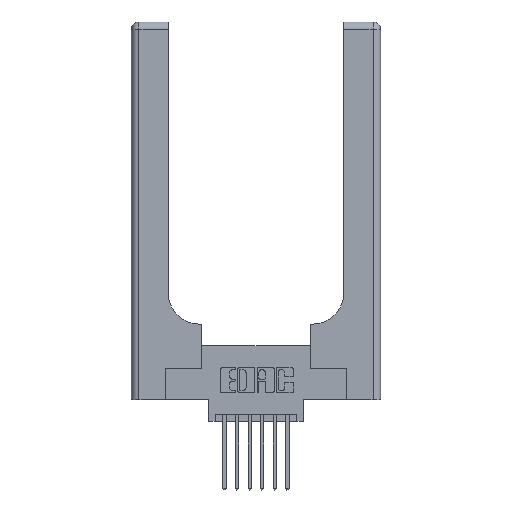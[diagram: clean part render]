
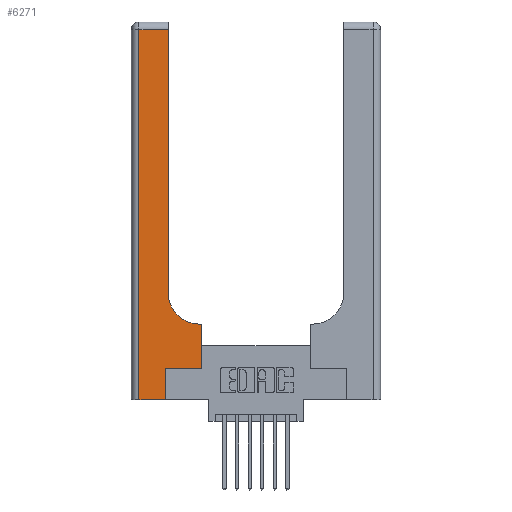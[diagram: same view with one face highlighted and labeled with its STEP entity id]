
A CAD part, top view. The second image highlights one B-rep face of the part: STEP entity #6271.
In plain terms, the highlighted planar face has unit normal (0, 0, 1).
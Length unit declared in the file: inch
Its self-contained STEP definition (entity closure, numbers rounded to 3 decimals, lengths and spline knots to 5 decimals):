
#11 = DIRECTION ( 'NONE',  ( -1., 0., 0. ) ) ;
#164 = VECTOR ( 'NONE', #244, 39.37008 ) ;
#244 = DIRECTION ( 'NONE',  ( 1., 0., 0. ) ) ;
#313 = CARTESIAN_POINT ( 'NONE',  ( 0.5415, 0.6, 0.37 ) ) ;
#494 = ORIENTED_EDGE ( 'NONE', *, *, #14081, .T. ) ;
#719 = VERTEX_POINT ( 'NONE', #2197 ) ;
#931 = CARTESIAN_POINT ( 'NONE',  ( 0.2915, 3., 0.37 ) ) ;
#1568 = DIRECTION ( 'NONE',  ( 0., -1., 0. ) ) ;
#2096 = EDGE_CURVE ( 'NONE', #6484, #9373, #3368, .T. ) ;
#2152 = ORIENTED_EDGE ( 'NONE', *, *, #4199, .T. ) ;
#2197 = CARTESIAN_POINT ( 'NONE',  ( 0.2915, 0.85, 0.37 ) ) ;
#2281 = VERTEX_POINT ( 'NONE', #12035 ) ;
#2461 = CARTESIAN_POINT ( 'NONE',  ( 0.2915, 2.94, 0.37 ) ) ;
#2558 = LINE ( 'NONE', #12146, #2929 ) ;
#2639 = CARTESIAN_POINT ( 'NONE',  ( 0., 2.94, 0.37 ) ) ;
#2873 = VERTEX_POINT ( 'NONE', #313 ) ;
#2910 = AXIS2_PLACEMENT_3D ( 'NONE', #7860, #9018, #4448 ) ;
#2929 = VECTOR ( 'NONE', #14321, 39.37008 ) ;
#3210 = EDGE_CURVE ( 'NONE', #9373, #6620, #13095, .T. ) ;
#3368 = LINE ( 'NONE', #6064, #164 ) ;
#3940 = EDGE_CURVE ( 'NONE', #719, #14530, #5670, .T. ) ;
#4199 = EDGE_CURVE ( 'NONE', #11435, #6484, #11259, .T. ) ;
#4448 = DIRECTION ( 'NONE',  ( 1., 0., 0. ) ) ;
#4592 = DIRECTION ( 'NONE',  ( 0., 0., -1. ) ) ;
#4832 = EDGE_CURVE ( 'NONE', #2281, #2873, #2558, .T. ) ;
#4838 = AXIS2_PLACEMENT_3D ( 'NONE', #5726, #4592, #11 ) ;
#4929 = VECTOR ( 'NONE', #8938, 39.37008 ) ;
#5104 = CARTESIAN_POINT ( 'NONE',  ( 0.269, 0.25, 0.37 ) ) ;
#5447 = FACE_OUTER_BOUND ( 'NONE', #13606, .T. ) ;
#5523 = DIRECTION ( 'NONE',  ( 1., 0., 0. ) ) ;
#5670 = LINE ( 'NONE', #931, #4929 ) ;
#5726 = CARTESIAN_POINT ( 'NONE',  ( 0., 3., 0.37 ) ) ;
#5857 = ORIENTED_EDGE ( 'NONE', *, *, #3940, .T. ) ;
#6064 = CARTESIAN_POINT ( 'NONE',  ( 0., 0., 0.37 ) ) ;
#6126 = VECTOR ( 'NONE', #14283, 39.37008 ) ;
#6271 = ADVANCED_FACE ( 'NONE', ( #5447 ), #12640, .F. ) ;
#6484 = VERTEX_POINT ( 'NONE', #9575 ) ;
#6620 = VERTEX_POINT ( 'NONE', #5104 ) ;
#6977 = ORIENTED_EDGE ( 'NONE', *, *, #8934, .T. ) ;
#7039 = EDGE_CURVE ( 'NONE', #2873, #719, #10347, .T. ) ;
#7147 = ORIENTED_EDGE ( 'NONE', *, *, #3210, .T. ) ;
#7860 = CARTESIAN_POINT ( 'NONE',  ( 0.5415, 0.85, 0.37 ) ) ;
#8168 = CARTESIAN_POINT ( 'NONE',  ( 0.06, 3., 0.37 ) ) ;
#8934 = EDGE_CURVE ( 'NONE', #6620, #11500, #12699, .T. ) ;
#8938 = DIRECTION ( 'NONE',  ( 0., 1., 0. ) ) ;
#9018 = DIRECTION ( 'NONE',  ( 0., 0., -1. ) ) ;
#9203 = CARTESIAN_POINT ( 'NONE',  ( 0.269, 0., 0.37 ) ) ;
#9305 = EDGE_CURVE ( 'NONE', #11500, #2281, #9426, .T. ) ;
#9373 = VERTEX_POINT ( 'NONE', #9203 ) ;
#9426 = LINE ( 'NONE', #11227, #11986 ) ;
#9429 = CARTESIAN_POINT ( 'NONE',  ( 0.06, 2.94, 0.37 ) ) ;
#9575 = CARTESIAN_POINT ( 'NONE',  ( 0.06, 0., 0.37 ) ) ;
#9622 = VECTOR ( 'NONE', #5523, 39.37008 ) ;
#10182 = CARTESIAN_POINT ( 'NONE',  ( 0.269, 0., 0.37 ) ) ;
#10347 = CIRCLE ( 'NONE', #2910, 0.25 ) ;
#10836 = ORIENTED_EDGE ( 'NONE', *, *, #7039, .T. ) ;
#10940 = ORIENTED_EDGE ( 'NONE', *, *, #2096, .T. ) ;
#11125 = VECTOR ( 'NONE', #14487, 39.37008 ) ;
#11192 = CARTESIAN_POINT ( 'NONE',  ( 0.5585, 0.25, 0.37 ) ) ;
#11227 = CARTESIAN_POINT ( 'NONE',  ( 0.5585, 0.25, 0.37 ) ) ;
#11259 = LINE ( 'NONE', #8168, #12356 ) ;
#11372 = DIRECTION ( 'NONE',  ( 0., 1., 0. ) ) ;
#11435 = VERTEX_POINT ( 'NONE', #9429 ) ;
#11500 = VERTEX_POINT ( 'NONE', #11192 ) ;
#11986 = VECTOR ( 'NONE', #11372, 39.37008 ) ;
#12035 = CARTESIAN_POINT ( 'NONE',  ( 0.5585, 0.6, 0.37 ) ) ;
#12146 = CARTESIAN_POINT ( 'NONE',  ( 0.2915, 0.6, 0.37 ) ) ;
#12356 = VECTOR ( 'NONE', #1568, 39.37008 ) ;
#12443 = CARTESIAN_POINT ( 'NONE',  ( 0.269, 0.25, 0.37 ) ) ;
#12640 = PLANE ( 'NONE',  #4838 ) ;
#12699 = LINE ( 'NONE', #12443, #9622 ) ;
#12810 = ORIENTED_EDGE ( 'NONE', *, *, #4832, .T. ) ;
#13095 = LINE ( 'NONE', #10182, #11125 ) ;
#13606 = EDGE_LOOP ( 'NONE', ( #5857, #494, #2152, #10940, #7147, #6977, #14790, #12810, #10836 ) ) ;
#14081 = EDGE_CURVE ( 'NONE', #14530, #11435, #14290, .T. ) ;
#14283 = DIRECTION ( 'NONE',  ( -1., 0., 0. ) ) ;
#14290 = LINE ( 'NONE', #2639, #6126 ) ;
#14321 = DIRECTION ( 'NONE',  ( -1., 0., 0. ) ) ;
#14487 = DIRECTION ( 'NONE',  ( 0., 1., 0. ) ) ;
#14530 = VERTEX_POINT ( 'NONE', #2461 ) ;
#14790 = ORIENTED_EDGE ( 'NONE', *, *, #9305, .T. ) ;
